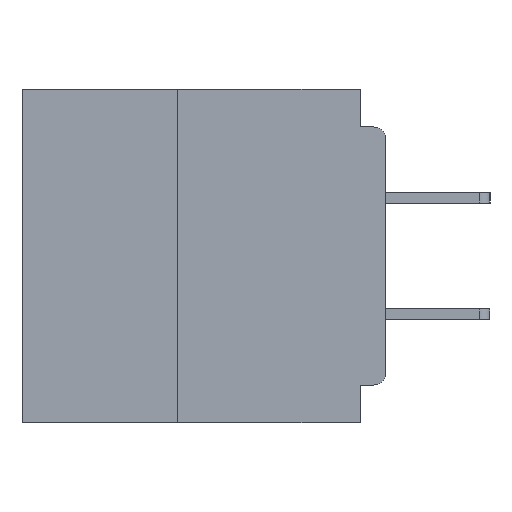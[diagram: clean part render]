
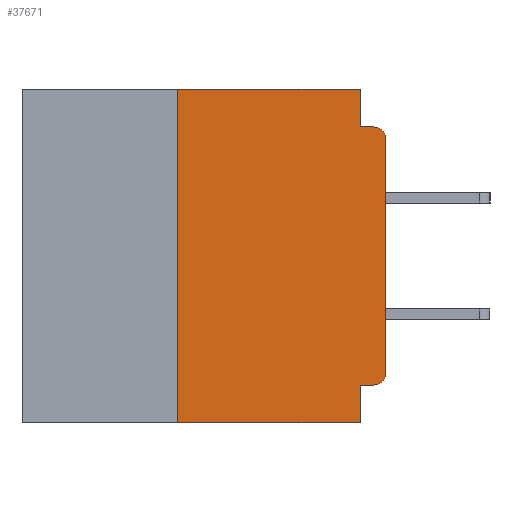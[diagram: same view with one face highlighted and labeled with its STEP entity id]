
A CAD part, left-side view. The second image highlights one B-rep face of the part: STEP entity #37671.
In plain terms, the highlighted planar face has unit normal (-1, 0, 0).
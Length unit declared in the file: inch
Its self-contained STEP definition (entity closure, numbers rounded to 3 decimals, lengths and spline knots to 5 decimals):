
#2452 = LINE ( 'NONE', #3692, #21784 ) ;
#2734 = EDGE_CURVE ( 'NONE', #9285, #7683, #46270, .T. ) ;
#2780 = VECTOR ( 'NONE', #50509, 39.37008 ) ;
#3565 = DIRECTION ( 'NONE',  ( 0., 0., 1. ) ) ;
#3692 = CARTESIAN_POINT ( 'NONE',  ( 0., 0.437, 0. ) ) ;
#4254 = LINE ( 'NONE', #12864, #2780 ) ;
#4849 = AXIS2_PLACEMENT_3D ( 'NONE', #46080, #17939, #50785 ) ;
#5576 = DIRECTION ( 'NONE',  ( 0., 0., -1. ) ) ;
#6069 = ORIENTED_EDGE ( 'NONE', *, *, #18647, .T. ) ;
#6509 = AXIS2_PLACEMENT_3D ( 'NONE', #57199, #33971, #5576 ) ;
#6537 = CARTESIAN_POINT ( 'NONE',  ( 0., 0.015, -0.06 ) ) ;
#7620 = VERTEX_POINT ( 'NONE', #28583 ) ;
#7683 = VERTEX_POINT ( 'NONE', #52484 ) ;
#8151 = DIRECTION ( 'NONE',  ( 0., 0., 1. ) ) ;
#8489 = DIRECTION ( 'NONE',  ( 0., -1., 0. ) ) ;
#9112 = EDGE_CURVE ( 'NONE', #22092, #45846, #45563, .T. ) ;
#9285 = VERTEX_POINT ( 'NONE', #18917 ) ;
#9739 = CARTESIAN_POINT ( 'NONE',  ( 0., 0., -0.355 ) ) ;
#11314 = DIRECTION ( 'NONE',  ( 0., 0., -1. ) ) ;
#12826 = EDGE_LOOP ( 'NONE', ( #37904, #22377, #24970, #49868, #55401, #29430, #6069, #59003, #42769, #29749 ) ) ;
#12864 = CARTESIAN_POINT ( 'NONE',  ( 0., 0.437, -0.4 ) ) ;
#12960 = DIRECTION ( 'NONE',  ( 0., 0., -1. ) ) ;
#16182 = EDGE_CURVE ( 'NONE', #26225, #7620, #32052, .T. ) ;
#16984 = CIRCLE ( 'NONE', #41877, 0.015 ) ;
#17939 = DIRECTION ( 'NONE',  ( -1., 0., 0. ) ) ;
#18017 = DIRECTION ( 'NONE',  ( 0., -1., 0. ) ) ;
#18630 = VERTEX_POINT ( 'NONE', #59650 ) ;
#18647 = EDGE_CURVE ( 'NONE', #22092, #59571, #4254, .T. ) ;
#18917 = CARTESIAN_POINT ( 'NONE',  ( 0., 0.031, 0. ) ) ;
#19372 = CARTESIAN_POINT ( 'NONE',  ( 0., 0.25, -0.4 ) ) ;
#19730 = PLANE ( 'NONE',  #6509 ) ;
#20550 = EDGE_CURVE ( 'NONE', #53339, #38508, #51045, .T. ) ;
#21784 = VECTOR ( 'NONE', #8489, 39.37008 ) ;
#21846 = EDGE_CURVE ( 'NONE', #7620, #59571, #27473, .T. ) ;
#22092 = VERTEX_POINT ( 'NONE', #19372 ) ;
#22377 = ORIENTED_EDGE ( 'NONE', *, *, #41453, .T. ) ;
#24970 = ORIENTED_EDGE ( 'NONE', *, *, #51994, .F. ) ;
#25659 = LINE ( 'NONE', #32106, #59958 ) ;
#26225 = VERTEX_POINT ( 'NONE', #44955 ) ;
#27473 = LINE ( 'NONE', #36517, #49417 ) ;
#28583 = CARTESIAN_POINT ( 'NONE',  ( 0., 0.031, -0.355 ) ) ;
#29430 = ORIENTED_EDGE ( 'NONE', *, *, #9112, .F. ) ;
#29504 = DIRECTION ( 'NONE',  ( 0., 0., -1. ) ) ;
#29749 = ORIENTED_EDGE ( 'NONE', *, *, #47726, .T. ) ;
#31784 = CARTESIAN_POINT ( 'NONE',  ( 0., 0., 0. ) ) ;
#32052 = LINE ( 'NONE', #9739, #44463 ) ;
#32106 = CARTESIAN_POINT ( 'NONE',  ( 0., 0., -0.045 ) ) ;
#33036 = CARTESIAN_POINT ( 'NONE',  ( 0., 0.031, 0. ) ) ;
#33157 = VECTOR ( 'NONE', #3565, 39.37008 ) ;
#33346 = DIRECTION ( 'NONE',  ( 0., 1., 0. ) ) ;
#33858 = VECTOR ( 'NONE', #29504, 39.37008 ) ;
#33969 = CARTESIAN_POINT ( 'NONE',  ( 0., 0.031, -0.4 ) ) ;
#33971 = DIRECTION ( 'NONE',  ( 1., 0., 0. ) ) ;
#36517 = CARTESIAN_POINT ( 'NONE',  ( 0., 0.031, -0.4 ) ) ;
#36667 = CARTESIAN_POINT ( 'NONE',  ( 0., 0.25, -0.4 ) ) ;
#37169 = VECTOR ( 'NONE', #8151, 39.37008 ) ;
#37652 = CARTESIAN_POINT ( 'NONE',  ( 0., 0., -0.34 ) ) ;
#37671 = ADVANCED_FACE ( 'NONE', ( #44211 ), #19730, .F. ) ;
#37904 = ORIENTED_EDGE ( 'NONE', *, *, #20550, .T. ) ;
#38508 = VERTEX_POINT ( 'NONE', #58731 ) ;
#39566 = DIRECTION ( 'NONE',  ( -1., 0., 0. ) ) ;
#41453 = EDGE_CURVE ( 'NONE', #38508, #18630, #16984, .T. ) ;
#41877 = AXIS2_PLACEMENT_3D ( 'NONE', #6537, #39566, #11314 ) ;
#42769 = ORIENTED_EDGE ( 'NONE', *, *, #16182, .F. ) ;
#44211 = FACE_OUTER_BOUND ( 'NONE', #12826, .T. ) ;
#44463 = VECTOR ( 'NONE', #33346, 39.37008 ) ;
#44955 = CARTESIAN_POINT ( 'NONE',  ( 0., 0.015, -0.355 ) ) ;
#45563 = LINE ( 'NONE', #36667, #33157 ) ;
#45846 = VERTEX_POINT ( 'NONE', #50578 ) ;
#46080 = CARTESIAN_POINT ( 'NONE',  ( 0., 0.015, -0.34 ) ) ;
#46270 = LINE ( 'NONE', #33036, #33858 ) ;
#47726 = EDGE_CURVE ( 'NONE', #26225, #53339, #60768, .T. ) ;
#49417 = VECTOR ( 'NONE', #12960, 39.37008 ) ;
#49868 = ORIENTED_EDGE ( 'NONE', *, *, #2734, .F. ) ;
#50509 = DIRECTION ( 'NONE',  ( 0., -1., 0. ) ) ;
#50578 = CARTESIAN_POINT ( 'NONE',  ( 0., 0.25, 0. ) ) ;
#50785 = DIRECTION ( 'NONE',  ( 0., 0., -1. ) ) ;
#51045 = LINE ( 'NONE', #31784, #37169 ) ;
#51994 = EDGE_CURVE ( 'NONE', #7683, #18630, #25659, .T. ) ;
#52484 = CARTESIAN_POINT ( 'NONE',  ( 0., 0.031, -0.045 ) ) ;
#53339 = VERTEX_POINT ( 'NONE', #37652 ) ;
#53767 = EDGE_CURVE ( 'NONE', #45846, #9285, #2452, .T. ) ;
#55401 = ORIENTED_EDGE ( 'NONE', *, *, #53767, .F. ) ;
#57199 = CARTESIAN_POINT ( 'NONE',  ( 0., 0.437, 0. ) ) ;
#58731 = CARTESIAN_POINT ( 'NONE',  ( 0., 0., -0.06 ) ) ;
#59003 = ORIENTED_EDGE ( 'NONE', *, *, #21846, .F. ) ;
#59571 = VERTEX_POINT ( 'NONE', #33969 ) ;
#59650 = CARTESIAN_POINT ( 'NONE',  ( 0., 0.015, -0.045 ) ) ;
#59958 = VECTOR ( 'NONE', #18017, 39.37008 ) ;
#60768 = CIRCLE ( 'NONE', #4849, 0.015 ) ;
